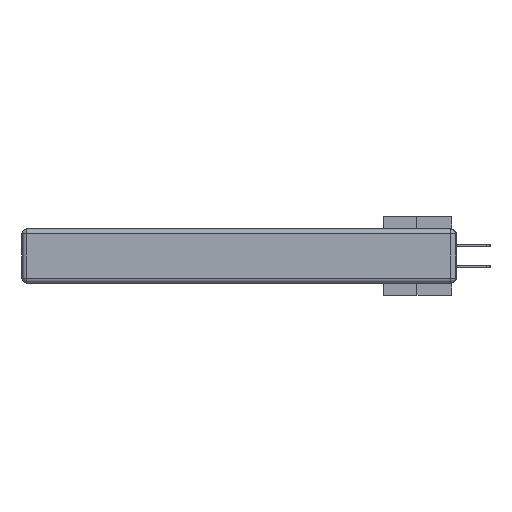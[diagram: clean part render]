
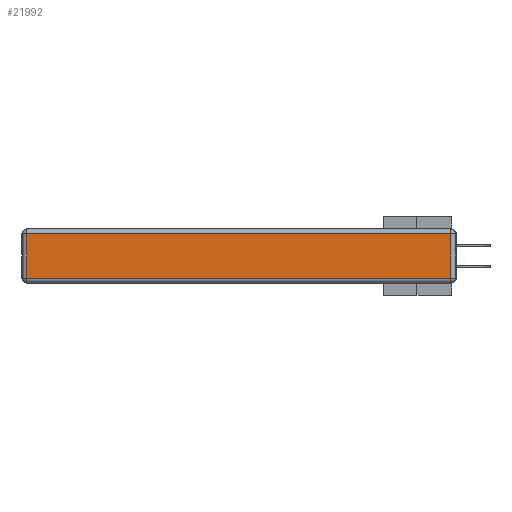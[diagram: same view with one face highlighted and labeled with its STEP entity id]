
A CAD part, left-side view. The second image highlights one B-rep face of the part: STEP entity #21992.
In plain terms, the highlighted planar face has unit normal (-1, 0, 0).
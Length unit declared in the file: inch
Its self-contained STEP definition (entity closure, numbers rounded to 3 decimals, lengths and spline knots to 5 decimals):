
#878 = VECTOR ( 'NONE', #36471, 39.37008 ) ;
#1353 = FACE_OUTER_BOUND ( 'NONE', #17979, .T. ) ;
#4415 = ORIENTED_EDGE ( 'NONE', *, *, #21279, .T. ) ;
#5328 = CARTESIAN_POINT ( 'NONE',  ( 0., 0.03, -0.313 ) ) ;
#5862 = VERTEX_POINT ( 'NONE', #35885 ) ;
#6627 = PLANE ( 'NONE',  #30565 ) ;
#8975 = CARTESIAN_POINT ( 'NONE',  ( 0., 0.03, -0.03 ) ) ;
#10154 = DIRECTION ( 'NONE',  ( -1., 0., 0. ) ) ;
#10778 = DIRECTION ( 'NONE',  ( 0., 0., 1. ) ) ;
#11612 = CARTESIAN_POINT ( 'NONE',  ( 0., 0., -0.313 ) ) ;
#12876 = CARTESIAN_POINT ( 'NONE',  ( 0., 2.75, -0.03 ) ) ;
#14988 = DIRECTION ( 'NONE',  ( 0., -1., 0. ) ) ;
#15188 = LINE ( 'NONE', #11612, #20645 ) ;
#16362 = EDGE_CURVE ( 'NONE', #25420, #39422, #45234, .T. ) ;
#16865 = EDGE_CURVE ( 'NONE', #5862, #25420, #15188, .T. ) ;
#17979 = EDGE_LOOP ( 'NONE', ( #37869, #39199, #4415, #28879 ) ) ;
#19727 = DIRECTION ( 'NONE',  ( 0., 0., 1. ) ) ;
#20645 = VECTOR ( 'NONE', #14988, 39.37008 ) ;
#21185 = EDGE_CURVE ( 'NONE', #42633, #5862, #23304, .T. ) ;
#21279 = EDGE_CURVE ( 'NONE', #39422, #42633, #26030, .T. ) ;
#21620 = CARTESIAN_POINT ( 'NONE',  ( 0., 2.72, -0.03 ) ) ;
#21992 = ADVANCED_FACE ( 'NONE', ( #1353 ), #6627, .T. ) ;
#23304 = LINE ( 'NONE', #40394, #878 ) ;
#25420 = VERTEX_POINT ( 'NONE', #5328 ) ;
#26030 = LINE ( 'NONE', #12876, #31487 ) ;
#28879 = ORIENTED_EDGE ( 'NONE', *, *, #21185, .T. ) ;
#30565 = AXIS2_PLACEMENT_3D ( 'NONE', #31093, #10154, #10778 ) ;
#31093 = CARTESIAN_POINT ( 'NONE',  ( 0., 0., -0.343 ) ) ;
#31487 = VECTOR ( 'NONE', #41112, 39.37008 ) ;
#35885 = CARTESIAN_POINT ( 'NONE',  ( 0., 2.72, -0.313 ) ) ;
#36471 = DIRECTION ( 'NONE',  ( 0., 0., -1. ) ) ;
#37068 = VECTOR ( 'NONE', #19727, 39.37008 ) ;
#37132 = CARTESIAN_POINT ( 'NONE',  ( 0., 0.03, -0.343 ) ) ;
#37869 = ORIENTED_EDGE ( 'NONE', *, *, #16865, .T. ) ;
#39199 = ORIENTED_EDGE ( 'NONE', *, *, #16362, .T. ) ;
#39422 = VERTEX_POINT ( 'NONE', #8975 ) ;
#40394 = CARTESIAN_POINT ( 'NONE',  ( 0., 2.72, -0.343 ) ) ;
#41112 = DIRECTION ( 'NONE',  ( 0., 1., 0. ) ) ;
#42633 = VERTEX_POINT ( 'NONE', #21620 ) ;
#45234 = LINE ( 'NONE', #37132, #37068 ) ;
